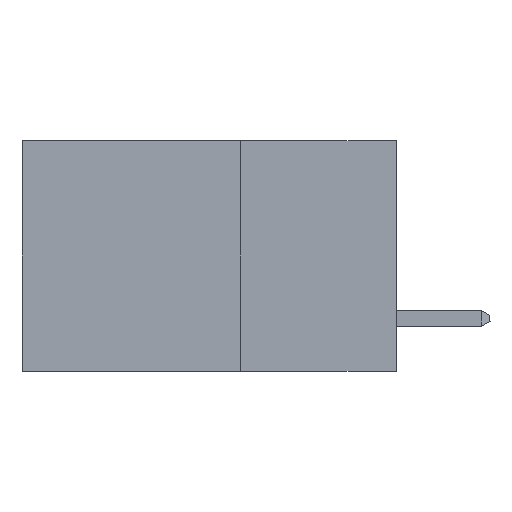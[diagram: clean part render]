
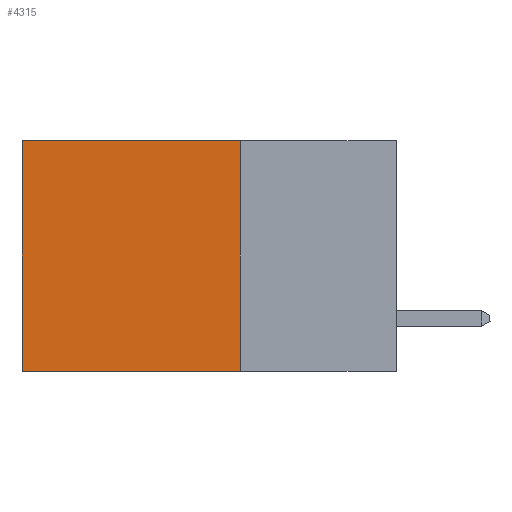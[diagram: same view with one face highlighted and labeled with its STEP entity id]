
A CAD part, left-side view. The second image highlights one B-rep face of the part: STEP entity #4315.
In plain terms, the highlighted planar face has unit normal (-1, 0, 0).
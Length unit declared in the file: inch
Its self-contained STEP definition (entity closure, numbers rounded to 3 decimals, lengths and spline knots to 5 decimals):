
#1276 = ORIENTED_EDGE ( 'NONE', *, *, #3965, .F. ) ;
#1666 = VERTEX_POINT ( 'NONE', #8761 ) ;
#2139 = AXIS2_PLACEMENT_3D ( 'NONE', #8735, #8804, #8785 ) ;
#2213 = LINE ( 'NONE', #12098, #12444 ) ;
#2268 = CARTESIAN_POINT ( 'NONE',  ( 0.298, 0.6, -0.37 ) ) ;
#2741 = VECTOR ( 'NONE', #8746, 39.37008 ) ;
#2823 = VECTOR ( 'NONE', #7547, 39.37008 ) ;
#2844 = FACE_OUTER_BOUND ( 'NONE', #4592, .T. ) ;
#2848 = VERTEX_POINT ( 'NONE', #7772 ) ;
#3064 = LINE ( 'NONE', #9743, #2741 ) ;
#3965 = EDGE_CURVE ( 'NONE', #2848, #1666, #2213, .T. ) ;
#4315 = ADVANCED_FACE ( 'NONE', ( #2844 ), #8830, .F. ) ;
#4592 = EDGE_LOOP ( 'NONE', ( #6074, #7278, #1276, #7764 ) ) ;
#6074 = ORIENTED_EDGE ( 'NONE', *, *, #12818, .T. ) ;
#6564 = CARTESIAN_POINT ( 'NONE',  ( 0.298, 0.25, 0. ) ) ;
#6640 = DIRECTION ( 'NONE',  ( 0., 0., -1. ) ) ;
#7278 = ORIENTED_EDGE ( 'NONE', *, *, #11520, .F. ) ;
#7314 = CARTESIAN_POINT ( 'NONE',  ( 0.298, 0.6, 0. ) ) ;
#7547 = DIRECTION ( 'NONE',  ( 0., 1., 0. ) ) ;
#7764 = ORIENTED_EDGE ( 'NONE', *, *, #9426, .T. ) ;
#7772 = CARTESIAN_POINT ( 'NONE',  ( 0.298, 0.25, 0. ) ) ;
#7964 = DIRECTION ( 'NONE',  ( 0., 0., -1. ) ) ;
#8735 = CARTESIAN_POINT ( 'NONE',  ( 0.298, 0.25, 0. ) ) ;
#8746 = DIRECTION ( 'NONE',  ( 0., 1., 0. ) ) ;
#8761 = CARTESIAN_POINT ( 'NONE',  ( 0.298, 0.25, -0.37 ) ) ;
#8785 = DIRECTION ( 'NONE',  ( 0., 0., -1. ) ) ;
#8804 = DIRECTION ( 'NONE',  ( 1., 0., 0. ) ) ;
#8830 = PLANE ( 'NONE',  #2139 ) ;
#9426 = EDGE_CURVE ( 'NONE', #2848, #9936, #10699, .T. ) ;
#9743 = CARTESIAN_POINT ( 'NONE',  ( 0.298, 0.25, -0.37 ) ) ;
#9936 = VERTEX_POINT ( 'NONE', #7314 ) ;
#10550 = VERTEX_POINT ( 'NONE', #2268 ) ;
#10699 = LINE ( 'NONE', #6564, #2823 ) ;
#11520 = EDGE_CURVE ( 'NONE', #1666, #10550, #3064, .T. ) ;
#11854 = VECTOR ( 'NONE', #6640, 39.37008 ) ;
#12098 = CARTESIAN_POINT ( 'NONE',  ( 0.298, 0.25, 0. ) ) ;
#12156 = LINE ( 'NONE', #12600, #11854 ) ;
#12444 = VECTOR ( 'NONE', #7964, 39.37008 ) ;
#12600 = CARTESIAN_POINT ( 'NONE',  ( 0.298, 0.6, 0. ) ) ;
#12818 = EDGE_CURVE ( 'NONE', #9936, #10550, #12156, .T. ) ;
